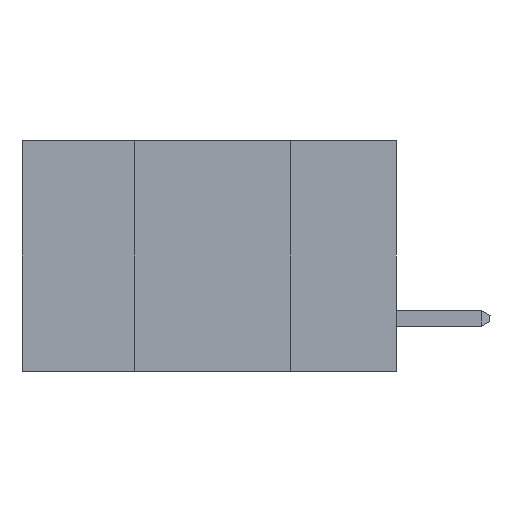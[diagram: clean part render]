
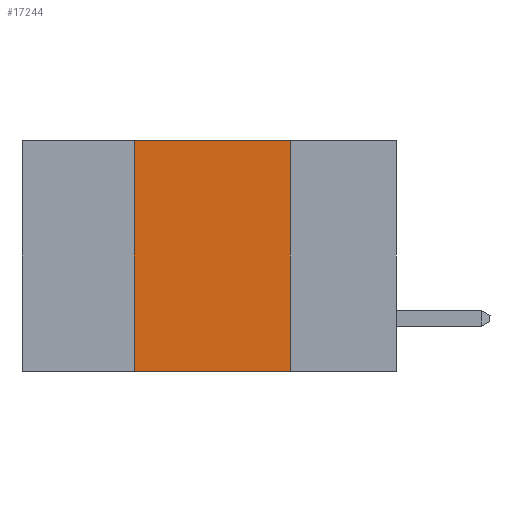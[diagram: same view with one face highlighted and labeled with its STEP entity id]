
A CAD part, left-side view. The second image highlights one B-rep face of the part: STEP entity #17244.
In plain terms, the highlighted planar face has unit normal (-1, 0, 0).
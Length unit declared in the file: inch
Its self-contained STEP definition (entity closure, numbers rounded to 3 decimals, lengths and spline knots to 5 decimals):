
#406 = DIRECTION ( 'NONE',  ( 0., 0., 1. ) ) ;
#3871 = EDGE_CURVE ( 'NONE', #30065, #29786, #11559, .T. ) ;
#5068 = CARTESIAN_POINT ( 'NONE',  ( 0., 0.6, 0. ) ) ;
#5378 = PLANE ( 'NONE',  #12406 ) ;
#5796 = ORIENTED_EDGE ( 'NONE', *, *, #5866, .F. ) ;
#5866 = EDGE_CURVE ( 'NONE', #29786, #22011, #19625, .T. ) ;
#7456 = LINE ( 'NONE', #18756, #24553 ) ;
#9212 = DIRECTION ( 'NONE',  ( 0., -1., 0. ) ) ;
#9954 = DIRECTION ( 'NONE',  ( 0., 0., -1. ) ) ;
#10535 = ORIENTED_EDGE ( 'NONE', *, *, #15488, .F. ) ;
#11261 = VERTEX_POINT ( 'NONE', #16290 ) ;
#11336 = LINE ( 'NONE', #29235, #25405 ) ;
#11559 = LINE ( 'NONE', #29059, #18609 ) ;
#12406 = AXIS2_PLACEMENT_3D ( 'NONE', #5068, #26427, #9954 ) ;
#13440 = EDGE_LOOP ( 'NONE', ( #10535, #5796, #21738, #17134 ) ) ;
#13473 = CARTESIAN_POINT ( 'NONE',  ( 0., 0.17, 0. ) ) ;
#15488 = EDGE_CURVE ( 'NONE', #22011, #11261, #11336, .T. ) ;
#16290 = CARTESIAN_POINT ( 'NONE',  ( 0., 0.17, -0.37 ) ) ;
#17134 = ORIENTED_EDGE ( 'NONE', *, *, #23160, .T. ) ;
#17244 = ADVANCED_FACE ( 'NONE', ( #26014 ), #5378, .F. ) ;
#18609 = VECTOR ( 'NONE', #406, 39.37008 ) ;
#18756 = CARTESIAN_POINT ( 'NONE',  ( 0., 0.6, -0.37 ) ) ;
#19461 = DIRECTION ( 'NONE',  ( 0., -1., 0. ) ) ;
#19625 = LINE ( 'NONE', #28779, #19988 ) ;
#19988 = VECTOR ( 'NONE', #19461, 39.37008 ) ;
#21465 = CARTESIAN_POINT ( 'NONE',  ( 0., 0.42, 0. ) ) ;
#21738 = ORIENTED_EDGE ( 'NONE', *, *, #3871, .F. ) ;
#22011 = VERTEX_POINT ( 'NONE', #13473 ) ;
#23160 = EDGE_CURVE ( 'NONE', #30065, #11261, #7456, .T. ) ;
#24553 = VECTOR ( 'NONE', #9212, 39.37008 ) ;
#25405 = VECTOR ( 'NONE', #28916, 39.37008 ) ;
#26014 = FACE_OUTER_BOUND ( 'NONE', #13440, .T. ) ;
#26427 = DIRECTION ( 'NONE',  ( 1., 0., 0. ) ) ;
#28033 = CARTESIAN_POINT ( 'NONE',  ( 0., 0.42, -0.37 ) ) ;
#28779 = CARTESIAN_POINT ( 'NONE',  ( 0., 0.6, 0. ) ) ;
#28916 = DIRECTION ( 'NONE',  ( 0., 0., -1. ) ) ;
#29059 = CARTESIAN_POINT ( 'NONE',  ( 0., 0.42, 0. ) ) ;
#29235 = CARTESIAN_POINT ( 'NONE',  ( 0., 0.17, 0. ) ) ;
#29786 = VERTEX_POINT ( 'NONE', #21465 ) ;
#30065 = VERTEX_POINT ( 'NONE', #28033 ) ;
